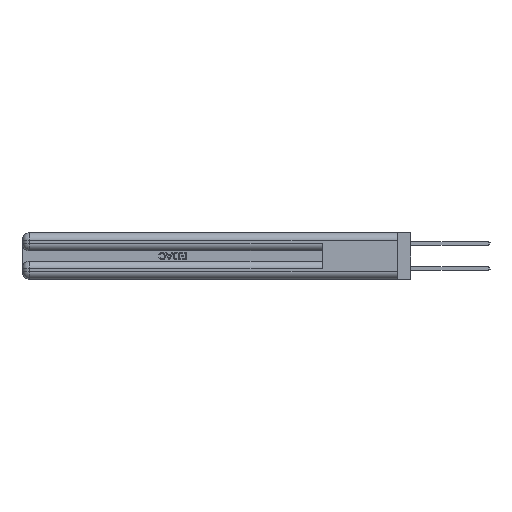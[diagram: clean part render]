
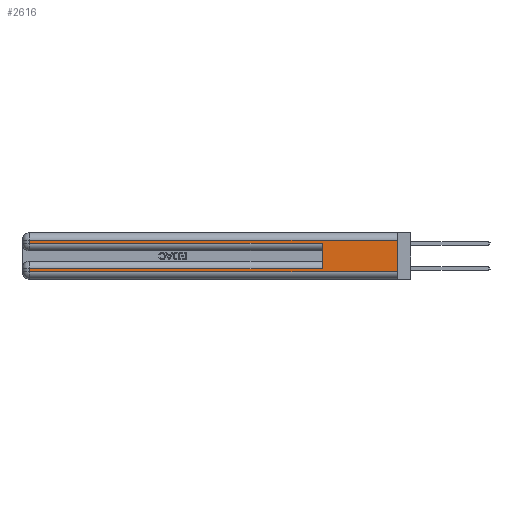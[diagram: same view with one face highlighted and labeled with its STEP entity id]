
A CAD part, left-side view. The second image highlights one B-rep face of the part: STEP entity #2616.
In plain terms, the highlighted planar face has unit normal (-1, 0, 0).
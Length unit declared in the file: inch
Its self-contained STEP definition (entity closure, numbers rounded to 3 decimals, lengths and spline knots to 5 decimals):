
#52 = EDGE_CURVE ( 'NONE', #3693, #36130, #33330, .T. ) ;
#211 = ORIENTED_EDGE ( 'NONE', *, *, #37533, .F. ) ;
#1359 = DIRECTION ( 'NONE',  ( 0., 0., -1. ) ) ;
#2142 = ORIENTED_EDGE ( 'NONE', *, *, #52, .T. ) ;
#2601 = EDGE_LOOP ( 'NONE', ( #211, #5366, #19886, #2142, #7308, #21805, #25588, #19934 ) ) ;
#2616 = ADVANCED_FACE ( 'NONE', ( #11813 ), #7522, .F. ) ;
#2915 = VERTEX_POINT ( 'NONE', #25092 ) ;
#3415 = CARTESIAN_POINT ( 'NONE',  ( 0., 0., 0.37 ) ) ;
#3693 = VERTEX_POINT ( 'NONE', #5282 ) ;
#3947 = DIRECTION ( 'NONE',  ( 0., 0., -1. ) ) ;
#4160 = EDGE_CURVE ( 'NONE', #26829, #36130, #16048, .T. ) ;
#5140 = LINE ( 'NONE', #23289, #35978 ) ;
#5282 = CARTESIAN_POINT ( 'NONE',  ( 0., 2.94, 0.285 ) ) ;
#5331 = CARTESIAN_POINT ( 'NONE',  ( 0., 2.94, 0.37 ) ) ;
#5366 = ORIENTED_EDGE ( 'NONE', *, *, #44695, .T. ) ;
#6482 = VECTOR ( 'NONE', #3947, 39.37008 ) ;
#6553 = VERTEX_POINT ( 'NONE', #49079 ) ;
#7308 = ORIENTED_EDGE ( 'NONE', *, *, #4160, .F. ) ;
#7522 = PLANE ( 'NONE',  #25693 ) ;
#9068 = DIRECTION ( 'NONE',  ( 0., -1., 0. ) ) ;
#10269 = CARTESIAN_POINT ( 'NONE',  ( 0., 0., 0.06 ) ) ;
#11620 = DIRECTION ( 'NONE',  ( 0., 0., -1. ) ) ;
#11813 = FACE_OUTER_BOUND ( 'NONE', #2601, .T. ) ;
#12019 = DIRECTION ( 'NONE',  ( 0., 0., 1. ) ) ;
#13023 = DIRECTION ( 'NONE',  ( 0., 1., 0. ) ) ;
#13863 = DIRECTION ( 'NONE',  ( 0., 1., 0. ) ) ;
#14083 = LINE ( 'NONE', #5331, #23472 ) ;
#15140 = VERTEX_POINT ( 'NONE', #44702 ) ;
#15260 = VERTEX_POINT ( 'NONE', #37377 ) ;
#15772 = CARTESIAN_POINT ( 'NONE',  ( 0., 0.6, 0.285 ) ) ;
#16048 = LINE ( 'NONE', #36019, #37347 ) ;
#17002 = EDGE_CURVE ( 'NONE', #26829, #15260, #30915, .T. ) ;
#17248 = LINE ( 'NONE', #32125, #6482 ) ;
#18308 = DIRECTION ( 'NONE',  ( 0., -1., 0. ) ) ;
#19854 = CARTESIAN_POINT ( 'NONE',  ( 0., 0., 0.06 ) ) ;
#19886 = ORIENTED_EDGE ( 'NONE', *, *, #28240, .T. ) ;
#19934 = ORIENTED_EDGE ( 'NONE', *, *, #44148, .T. ) ;
#20254 = VECTOR ( 'NONE', #13023, 39.37008 ) ;
#20902 = CARTESIAN_POINT ( 'NONE',  ( 0., 0., 0.085 ) ) ;
#21805 = ORIENTED_EDGE ( 'NONE', *, *, #17002, .T. ) ;
#23289 = CARTESIAN_POINT ( 'NONE',  ( 0., 2.94, 0.37 ) ) ;
#23472 = VECTOR ( 'NONE', #1359, 39.37008 ) ;
#25092 = CARTESIAN_POINT ( 'NONE',  ( 0., 2.94, 0.06 ) ) ;
#25588 = ORIENTED_EDGE ( 'NONE', *, *, #37802, .T. ) ;
#25693 = AXIS2_PLACEMENT_3D ( 'NONE', #3415, #39485, #11620 ) ;
#26829 = VERTEX_POINT ( 'NONE', #27101 ) ;
#27101 = CARTESIAN_POINT ( 'NONE',  ( 0., 0.6, 0.085 ) ) ;
#28240 = EDGE_CURVE ( 'NONE', #15140, #3693, #5140, .T. ) ;
#28671 = LINE ( 'NONE', #33880, #40574 ) ;
#30915 = LINE ( 'NONE', #20902, #20254 ) ;
#32125 = CARTESIAN_POINT ( 'NONE',  ( 0., 0., 0.37 ) ) ;
#32496 = LINE ( 'NONE', #10269, #43080 ) ;
#33118 = CARTESIAN_POINT ( 'NONE',  ( 0., 0., 0.285 ) ) ;
#33330 = LINE ( 'NONE', #33118, #35827 ) ;
#33880 = CARTESIAN_POINT ( 'NONE',  ( 0., 0., 0.31 ) ) ;
#35827 = VECTOR ( 'NONE', #9068, 39.37008 ) ;
#35978 = VECTOR ( 'NONE', #47213, 39.37008 ) ;
#36019 = CARTESIAN_POINT ( 'NONE',  ( 0., 0.6, 0.145 ) ) ;
#36130 = VERTEX_POINT ( 'NONE', #15772 ) ;
#37347 = VECTOR ( 'NONE', #12019, 39.37008 ) ;
#37377 = CARTESIAN_POINT ( 'NONE',  ( 0., 2.94, 0.085 ) ) ;
#37533 = EDGE_CURVE ( 'NONE', #6553, #40604, #17248, .T. ) ;
#37802 = EDGE_CURVE ( 'NONE', #15260, #2915, #14083, .T. ) ;
#39485 = DIRECTION ( 'NONE',  ( 1., 0., 0. ) ) ;
#40574 = VECTOR ( 'NONE', #13863, 39.37008 ) ;
#40604 = VERTEX_POINT ( 'NONE', #19854 ) ;
#43080 = VECTOR ( 'NONE', #18308, 39.37008 ) ;
#44148 = EDGE_CURVE ( 'NONE', #2915, #40604, #32496, .T. ) ;
#44695 = EDGE_CURVE ( 'NONE', #6553, #15140, #28671, .T. ) ;
#44702 = CARTESIAN_POINT ( 'NONE',  ( 0., 2.94, 0.31 ) ) ;
#47213 = DIRECTION ( 'NONE',  ( 0., 0., -1. ) ) ;
#49079 = CARTESIAN_POINT ( 'NONE',  ( 0., 0., 0.31 ) ) ;
